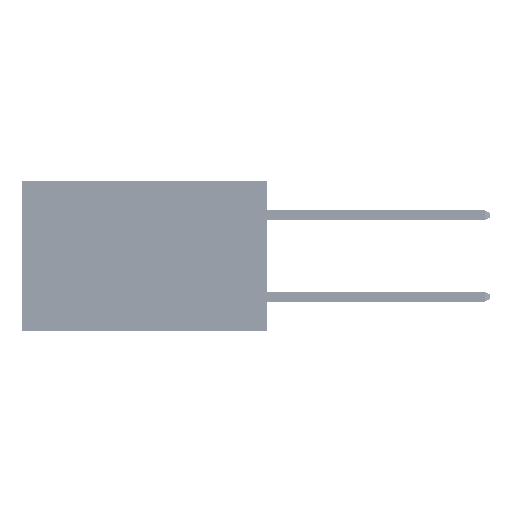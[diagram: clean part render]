
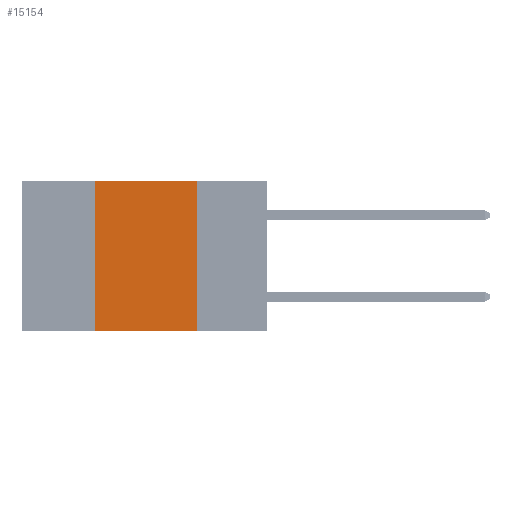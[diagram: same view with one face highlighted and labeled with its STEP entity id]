
A CAD part, left-side view. The second image highlights one B-rep face of the part: STEP entity #15154.
In plain terms, the highlighted planar face has unit normal (-1, 0, 0).
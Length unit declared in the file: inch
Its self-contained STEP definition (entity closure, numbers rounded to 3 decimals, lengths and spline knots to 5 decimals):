
#699 = VECTOR ( 'NONE', #38437, 39.37008 ) ;
#3374 = EDGE_CURVE ( 'NONE', #19686, #8167, #50061, .T. ) ;
#6877 = DIRECTION ( 'NONE',  ( 0., 0., -1. ) ) ;
#7880 = VECTOR ( 'NONE', #23958, 39.37008 ) ;
#8167 = VERTEX_POINT ( 'NONE', #49095 ) ;
#8730 = AXIS2_PLACEMENT_3D ( 'NONE', #51445, #39284, #6877 ) ;
#10503 = DIRECTION ( 'NONE',  ( 0., -1., 0. ) ) ;
#11424 = EDGE_CURVE ( 'NONE', #30184, #8167, #36366, .T. ) ;
#11442 = VERTEX_POINT ( 'NONE', #16007 ) ;
#11574 = CARTESIAN_POINT ( 'NONE',  ( 0., 0.17, 0. ) ) ;
#13214 = VECTOR ( 'NONE', #32660, 39.37008 ) ;
#15154 = ADVANCED_FACE ( 'NONE', ( #29823 ), #26732, .F. ) ;
#16007 = CARTESIAN_POINT ( 'NONE',  ( 0., 0.42, 0. ) ) ;
#19686 = VERTEX_POINT ( 'NONE', #28008 ) ;
#20557 = VECTOR ( 'NONE', #10503, 39.37008 ) ;
#23323 = EDGE_LOOP ( 'NONE', ( #50516, #36947, #27618, #49601 ) ) ;
#23785 = CARTESIAN_POINT ( 'NONE',  ( 0., 0.17, 0. ) ) ;
#23958 = DIRECTION ( 'NONE',  ( 0., 0., -1. ) ) ;
#26732 = PLANE ( 'NONE',  #8730 ) ;
#27531 = CARTESIAN_POINT ( 'NONE',  ( 0., 0.6, -0.37 ) ) ;
#27618 = ORIENTED_EDGE ( 'NONE', *, *, #41496, .F. ) ;
#28008 = CARTESIAN_POINT ( 'NONE',  ( 0., 0.42, -0.37 ) ) ;
#29823 = FACE_OUTER_BOUND ( 'NONE', #23323, .T. ) ;
#30184 = VERTEX_POINT ( 'NONE', #23785 ) ;
#30550 = CARTESIAN_POINT ( 'NONE',  ( 0., 0.6, 0. ) ) ;
#32660 = DIRECTION ( 'NONE',  ( 0., -1., 0. ) ) ;
#36366 = LINE ( 'NONE', #11574, #7880 ) ;
#36947 = ORIENTED_EDGE ( 'NONE', *, *, #44462, .F. ) ;
#38437 = DIRECTION ( 'NONE',  ( 0., 0., 1. ) ) ;
#39284 = DIRECTION ( 'NONE',  ( 1., 0., 0. ) ) ;
#40243 = LINE ( 'NONE', #30550, #20557 ) ;
#40698 = LINE ( 'NONE', #46138, #699 ) ;
#41496 = EDGE_CURVE ( 'NONE', #19686, #11442, #40698, .T. ) ;
#44462 = EDGE_CURVE ( 'NONE', #11442, #30184, #40243, .T. ) ;
#46138 = CARTESIAN_POINT ( 'NONE',  ( 0., 0.42, 0. ) ) ;
#49095 = CARTESIAN_POINT ( 'NONE',  ( 0., 0.17, -0.37 ) ) ;
#49601 = ORIENTED_EDGE ( 'NONE', *, *, #3374, .T. ) ;
#50061 = LINE ( 'NONE', #27531, #13214 ) ;
#50516 = ORIENTED_EDGE ( 'NONE', *, *, #11424, .F. ) ;
#51445 = CARTESIAN_POINT ( 'NONE',  ( 0., 0.6, 0. ) ) ;
